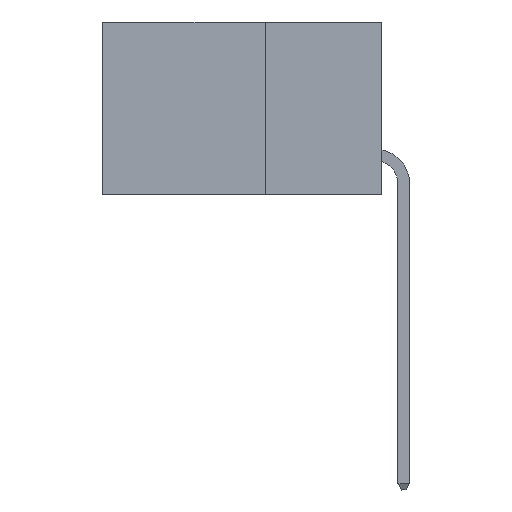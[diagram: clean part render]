
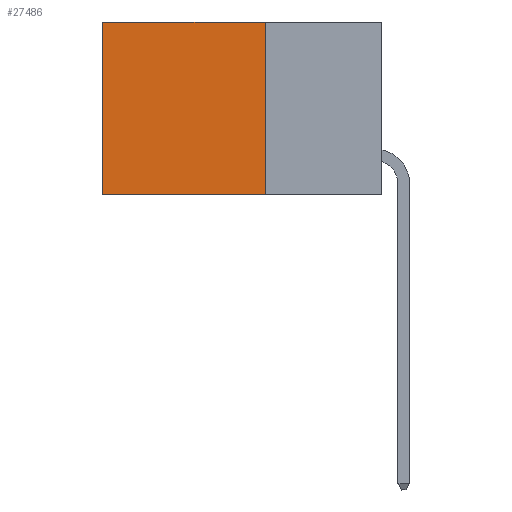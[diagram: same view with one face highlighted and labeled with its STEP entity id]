
A CAD part, left-side view. The second image highlights one B-rep face of the part: STEP entity #27486.
In plain terms, the highlighted planar face has unit normal (-1, 0, 0).
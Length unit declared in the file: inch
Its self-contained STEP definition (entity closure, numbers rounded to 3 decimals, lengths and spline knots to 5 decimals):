
#3761 = VERTEX_POINT ( 'NONE', #28895 ) ;
#5429 = CARTESIAN_POINT ( 'NONE',  ( 0.2875, 0.25, 0. ) ) ;
#5596 = VERTEX_POINT ( 'NONE', #30049 ) ;
#6135 = PLANE ( 'NONE',  #25051 ) ;
#9791 = VECTOR ( 'NONE', #22340, 39.37008 ) ;
#11810 = LINE ( 'NONE', #22046, #42205 ) ;
#12664 = EDGE_CURVE ( 'NONE', #19919, #5596, #31451, .T. ) ;
#12968 = VERTEX_POINT ( 'NONE', #34318 ) ;
#13192 = CARTESIAN_POINT ( 'NONE',  ( 0.2875, 0.25, -0.37 ) ) ;
#13510 = FACE_OUTER_BOUND ( 'NONE', #41619, .T. ) ;
#13703 = EDGE_CURVE ( 'NONE', #19919, #3761, #13831, .T. ) ;
#13831 = LINE ( 'NONE', #38417, #28231 ) ;
#14581 = DIRECTION ( 'NONE',  ( 0., 0., -1. ) ) ;
#14832 = CARTESIAN_POINT ( 'NONE',  ( 0.2875, 0.25, 0. ) ) ;
#17076 = ORIENTED_EDGE ( 'NONE', *, *, #13703, .F. ) ;
#19919 = VERTEX_POINT ( 'NONE', #5429 ) ;
#22046 = CARTESIAN_POINT ( 'NONE',  ( 0.2875, 0.6, 0. ) ) ;
#22340 = DIRECTION ( 'NONE',  ( 0., 1., 0. ) ) ;
#22389 = ORIENTED_EDGE ( 'NONE', *, *, #27659, .T. ) ;
#24517 = VECTOR ( 'NONE', #35441, 39.37008 ) ;
#24708 = DIRECTION ( 'NONE',  ( 0., 0., -1. ) ) ;
#25051 = AXIS2_PLACEMENT_3D ( 'NONE', #29959, #29821, #26694 ) ;
#26694 = DIRECTION ( 'NONE',  ( 0., 0., -1. ) ) ;
#27486 = ADVANCED_FACE ( 'NONE', ( #13510 ), #6135, .F. ) ;
#27659 = EDGE_CURVE ( 'NONE', #5596, #12968, #11810, .T. ) ;
#28231 = VECTOR ( 'NONE', #24708, 39.37008 ) ;
#28459 = ORIENTED_EDGE ( 'NONE', *, *, #12664, .T. ) ;
#28895 = CARTESIAN_POINT ( 'NONE',  ( 0.2875, 0.25, -0.37 ) ) ;
#29821 = DIRECTION ( 'NONE',  ( 1., 0., 0. ) ) ;
#29959 = CARTESIAN_POINT ( 'NONE',  ( 0.2875, 0.25, 0. ) ) ;
#30049 = CARTESIAN_POINT ( 'NONE',  ( 0.2875, 0.6, 0. ) ) ;
#31451 = LINE ( 'NONE', #14832, #24517 ) ;
#31468 = EDGE_CURVE ( 'NONE', #3761, #12968, #32185, .T. ) ;
#32185 = LINE ( 'NONE', #13192, #9791 ) ;
#32921 = ORIENTED_EDGE ( 'NONE', *, *, #31468, .F. ) ;
#34318 = CARTESIAN_POINT ( 'NONE',  ( 0.2875, 0.6, -0.37 ) ) ;
#35441 = DIRECTION ( 'NONE',  ( 0., 1., 0. ) ) ;
#38417 = CARTESIAN_POINT ( 'NONE',  ( 0.2875, 0.25, 0. ) ) ;
#41619 = EDGE_LOOP ( 'NONE', ( #22389, #32921, #17076, #28459 ) ) ;
#42205 = VECTOR ( 'NONE', #14581, 39.37008 ) ;
